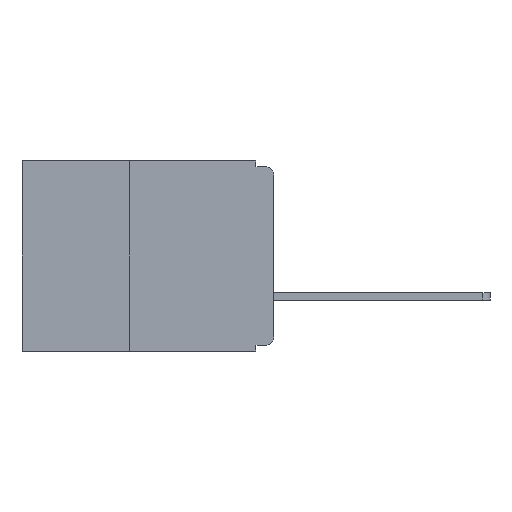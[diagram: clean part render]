
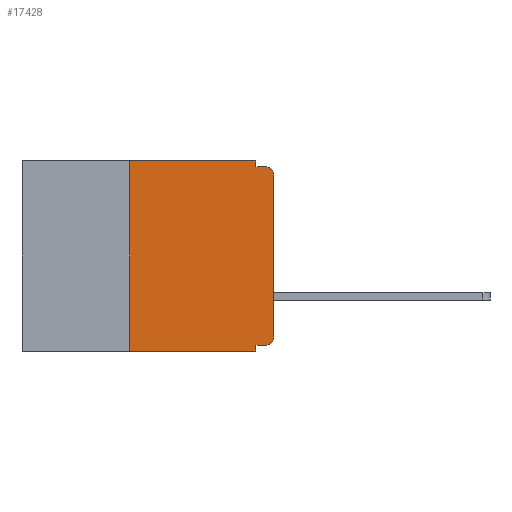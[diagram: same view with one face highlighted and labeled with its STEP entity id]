
A CAD part, left-side view. The second image highlights one B-rep face of the part: STEP entity #17428.
In plain terms, the highlighted planar face has unit normal (-1, 0, 0).
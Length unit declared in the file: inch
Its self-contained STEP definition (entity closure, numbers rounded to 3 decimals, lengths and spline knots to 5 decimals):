
#17 = LINE ( 'NONE', #27287, #25643 ) ;
#445 = ORIENTED_EDGE ( 'NONE', *, *, #14116, .F. ) ;
#751 = CARTESIAN_POINT ( 'NONE',  ( 0., 0.015, -0.025 ) ) ;
#1417 = CARTESIAN_POINT ( 'NONE',  ( 0., 0., -0.32 ) ) ;
#1467 = ORIENTED_EDGE ( 'NONE', *, *, #7172, .T. ) ;
#1569 = CARTESIAN_POINT ( 'NONE',  ( 0., 0.437, 0. ) ) ;
#1776 = ORIENTED_EDGE ( 'NONE', *, *, #13969, .T. ) ;
#2538 = CARTESIAN_POINT ( 'NONE',  ( 0., 0.25, -0.33 ) ) ;
#3183 = VERTEX_POINT ( 'NONE', #18402 ) ;
#3240 = DIRECTION ( 'NONE',  ( 0., 0., -1. ) ) ;
#3947 = EDGE_CURVE ( 'NONE', #15015, #4448, #27979, .T. ) ;
#4054 = DIRECTION ( 'NONE',  ( 0., 0., -1. ) ) ;
#4375 = LINE ( 'NONE', #9446, #16955 ) ;
#4448 = VERTEX_POINT ( 'NONE', #20392 ) ;
#4558 = ORIENTED_EDGE ( 'NONE', *, *, #5184, .F. ) ;
#5107 = VECTOR ( 'NONE', #23864, 39.37008 ) ;
#5184 = EDGE_CURVE ( 'NONE', #20401, #19579, #4375, .T. ) ;
#5873 = DIRECTION ( 'NONE',  ( -1., 0., 0. ) ) ;
#6506 = CARTESIAN_POINT ( 'NONE',  ( 0., 0.031, -0.32 ) ) ;
#6511 = CARTESIAN_POINT ( 'NONE',  ( 0., 0.437, 0. ) ) ;
#7172 = EDGE_CURVE ( 'NONE', #27577, #10439, #10138, .T. ) ;
#7642 = VECTOR ( 'NONE', #10691, 39.37008 ) ;
#7673 = DIRECTION ( 'NONE',  ( 0., -1., 0. ) ) ;
#8105 = VECTOR ( 'NONE', #19123, 39.37008 ) ;
#8269 = EDGE_CURVE ( 'NONE', #4448, #3183, #27738, .T. ) ;
#9207 = CARTESIAN_POINT ( 'NONE',  ( 0., 0., -0.025 ) ) ;
#9346 = CARTESIAN_POINT ( 'NONE',  ( 0., 0.015, -0.01 ) ) ;
#9446 = CARTESIAN_POINT ( 'NONE',  ( 0., 0.031, -0.33 ) ) ;
#9562 = DIRECTION ( 'NONE',  ( 0., 0., -1. ) ) ;
#9798 = LINE ( 'NONE', #21143, #15675 ) ;
#10138 = LINE ( 'NONE', #22196, #22613 ) ;
#10439 = VERTEX_POINT ( 'NONE', #9207 ) ;
#10649 = CARTESIAN_POINT ( 'NONE',  ( 0., 0.031, -0.33 ) ) ;
#10656 = CIRCLE ( 'NONE', #19149, 0.015 ) ;
#10691 = DIRECTION ( 'NONE',  ( 0., -1., 0. ) ) ;
#11197 = AXIS2_PLACEMENT_3D ( 'NONE', #751, #18259, #3240 ) ;
#11558 = ORIENTED_EDGE ( 'NONE', *, *, #19074, .F. ) ;
#12090 = VERTEX_POINT ( 'NONE', #20595 ) ;
#13491 = VERTEX_POINT ( 'NONE', #31021 ) ;
#13755 = DIRECTION ( 'NONE',  ( 0., 0., -1. ) ) ;
#13784 = CIRCLE ( 'NONE', #11197, 0.015 ) ;
#13969 = EDGE_CURVE ( 'NONE', #12090, #27577, #10656, .T. ) ;
#14116 = EDGE_CURVE ( 'NONE', #12090, #20401, #31249, .T. ) ;
#15015 = VERTEX_POINT ( 'NONE', #2538 ) ;
#15675 = VECTOR ( 'NONE', #13755, 39.37008 ) ;
#16601 = VECTOR ( 'NONE', #28075, 39.37008 ) ;
#16697 = AXIS2_PLACEMENT_3D ( 'NONE', #1569, #19080, #4054 ) ;
#16712 = FACE_OUTER_BOUND ( 'NONE', #22077, .T. ) ;
#16955 = VECTOR ( 'NONE', #9562, 39.37008 ) ;
#17215 = DIRECTION ( 'NONE',  ( 0., 0., 1. ) ) ;
#17428 = ADVANCED_FACE ( 'NONE', ( #16712 ), #26306, .F. ) ;
#18121 = CARTESIAN_POINT ( 'NONE',  ( 0., 0.437, -0.33 ) ) ;
#18259 = DIRECTION ( 'NONE',  ( -1., 0., 0. ) ) ;
#18402 = CARTESIAN_POINT ( 'NONE',  ( 0., 0.031, 0. ) ) ;
#19074 = EDGE_CURVE ( 'NONE', #3183, #13491, #9798, .T. ) ;
#19080 = DIRECTION ( 'NONE',  ( 1., 0., 0. ) ) ;
#19123 = DIRECTION ( 'NONE',  ( 0., -1., 0. ) ) ;
#19149 = AXIS2_PLACEMENT_3D ( 'NONE', #20878, #5873, #23350 ) ;
#19446 = ORIENTED_EDGE ( 'NONE', *, *, #8269, .F. ) ;
#19550 = ORIENTED_EDGE ( 'NONE', *, *, #26203, .T. ) ;
#19579 = VERTEX_POINT ( 'NONE', #10649 ) ;
#20392 = CARTESIAN_POINT ( 'NONE',  ( 0., 0.25, 0. ) ) ;
#20401 = VERTEX_POINT ( 'NONE', #6506 ) ;
#20595 = CARTESIAN_POINT ( 'NONE',  ( 0., 0.015, -0.32 ) ) ;
#20878 = CARTESIAN_POINT ( 'NONE',  ( 0., 0.015, -0.305 ) ) ;
#21143 = CARTESIAN_POINT ( 'NONE',  ( 0., 0.031, 0. ) ) ;
#22077 = EDGE_LOOP ( 'NONE', ( #1467, #23482, #26435, #11558, #19446, #30629, #19550, #4558, #445, #1776 ) ) ;
#22196 = CARTESIAN_POINT ( 'NONE',  ( 0., 0., 0. ) ) ;
#22478 = LINE ( 'NONE', #18121, #7642 ) ;
#22613 = VECTOR ( 'NONE', #17215, 39.37008 ) ;
#23350 = DIRECTION ( 'NONE',  ( 0., 0., -1. ) ) ;
#23482 = ORIENTED_EDGE ( 'NONE', *, *, #23904, .T. ) ;
#23864 = DIRECTION ( 'NONE',  ( 0., 1., 0. ) ) ;
#23904 = EDGE_CURVE ( 'NONE', #10439, #26536, #13784, .T. ) ;
#25643 = VECTOR ( 'NONE', #7673, 39.37008 ) ;
#26203 = EDGE_CURVE ( 'NONE', #15015, #19579, #22478, .T. ) ;
#26306 = PLANE ( 'NONE',  #16697 ) ;
#26435 = ORIENTED_EDGE ( 'NONE', *, *, #29758, .F. ) ;
#26536 = VERTEX_POINT ( 'NONE', #9346 ) ;
#26618 = CARTESIAN_POINT ( 'NONE',  ( 0., 0., -0.305 ) ) ;
#27287 = CARTESIAN_POINT ( 'NONE',  ( 0., 0., -0.01 ) ) ;
#27577 = VERTEX_POINT ( 'NONE', #26618 ) ;
#27738 = LINE ( 'NONE', #6511, #8105 ) ;
#27979 = LINE ( 'NONE', #28156, #16601 ) ;
#28075 = DIRECTION ( 'NONE',  ( 0., 0., 1. ) ) ;
#28156 = CARTESIAN_POINT ( 'NONE',  ( 0., 0.25, -0.33 ) ) ;
#29758 = EDGE_CURVE ( 'NONE', #13491, #26536, #17, .T. ) ;
#30629 = ORIENTED_EDGE ( 'NONE', *, *, #3947, .F. ) ;
#31021 = CARTESIAN_POINT ( 'NONE',  ( 0., 0.031, -0.01 ) ) ;
#31249 = LINE ( 'NONE', #1417, #5107 ) ;
